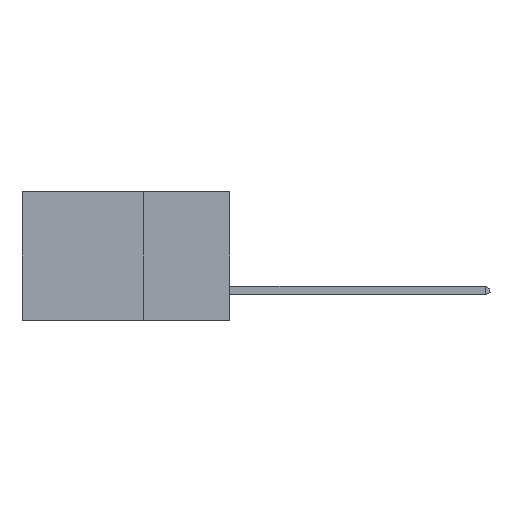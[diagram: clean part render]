
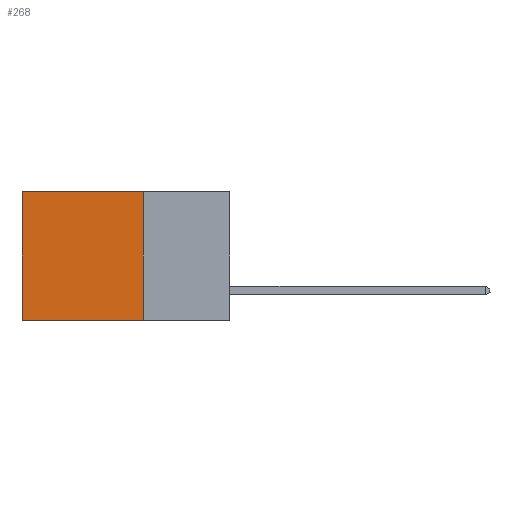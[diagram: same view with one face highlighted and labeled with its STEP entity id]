
A CAD part, left-side view. The second image highlights one B-rep face of the part: STEP entity #268.
In plain terms, the highlighted planar face has unit normal (-1, 0, 0).
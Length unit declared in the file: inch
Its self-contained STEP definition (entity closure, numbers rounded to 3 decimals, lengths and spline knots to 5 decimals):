
#268 = ADVANCED_FACE ( 'NONE', ( #10347 ), #14118, .F. ) ;
#783 = CARTESIAN_POINT ( 'NONE',  ( 0.298, 0.25, -0.37 ) ) ;
#1923 = CARTESIAN_POINT ( 'NONE',  ( 0.298, 0.6, 0. ) ) ;
#2103 = EDGE_CURVE ( 'NONE', #6059, #18060, #12095, .T. ) ;
#2586 = ORIENTED_EDGE ( 'NONE', *, *, #2103, .F. ) ;
#3015 = AXIS2_PLACEMENT_3D ( 'NONE', #20912, #3309, #9962 ) ;
#3309 = DIRECTION ( 'NONE',  ( 1., 0., 0. ) ) ;
#5392 = LINE ( 'NONE', #783, #20162 ) ;
#5785 = VERTEX_POINT ( 'NONE', #20310 ) ;
#6059 = VERTEX_POINT ( 'NONE', #13394 ) ;
#6519 = CARTESIAN_POINT ( 'NONE',  ( 0.298, 0.25, 0. ) ) ;
#6719 = CARTESIAN_POINT ( 'NONE',  ( 0.298, 0.25, 0. ) ) ;
#6841 = LINE ( 'NONE', #1923, #18785 ) ;
#9962 = DIRECTION ( 'NONE',  ( 0., 0., -1. ) ) ;
#10347 = FACE_OUTER_BOUND ( 'NONE', #27989, .T. ) ;
#10906 = ORIENTED_EDGE ( 'NONE', *, *, #12861, .F. ) ;
#12095 = LINE ( 'NONE', #6719, #21384 ) ;
#12435 = ORIENTED_EDGE ( 'NONE', *, *, #14252, .T. ) ;
#12861 = EDGE_CURVE ( 'NONE', #18060, #5785, #5392, .T. ) ;
#13394 = CARTESIAN_POINT ( 'NONE',  ( 0.298, 0.25, 0. ) ) ;
#13502 = CARTESIAN_POINT ( 'NONE',  ( 0.298, 0.25, -0.37 ) ) ;
#14118 = PLANE ( 'NONE',  #3015 ) ;
#14252 = EDGE_CURVE ( 'NONE', #6059, #21270, #27258, .T. ) ;
#14572 = CARTESIAN_POINT ( 'NONE',  ( 0.298, 0.6, 0. ) ) ;
#17313 = DIRECTION ( 'NONE',  ( 0., 0., -1. ) ) ;
#17530 = DIRECTION ( 'NONE',  ( 0., 0., -1. ) ) ;
#17904 = EDGE_CURVE ( 'NONE', #21270, #5785, #6841, .T. ) ;
#18060 = VERTEX_POINT ( 'NONE', #13502 ) ;
#18394 = DIRECTION ( 'NONE',  ( 0., 1., 0. ) ) ;
#18785 = VECTOR ( 'NONE', #17313, 39.37008 ) ;
#20162 = VECTOR ( 'NONE', #18394, 39.37008 ) ;
#20310 = CARTESIAN_POINT ( 'NONE',  ( 0.298, 0.6, -0.37 ) ) ;
#20912 = CARTESIAN_POINT ( 'NONE',  ( 0.298, 0.25, 0. ) ) ;
#21270 = VERTEX_POINT ( 'NONE', #14572 ) ;
#21384 = VECTOR ( 'NONE', #17530, 39.37008 ) ;
#25517 = ORIENTED_EDGE ( 'NONE', *, *, #17904, .T. ) ;
#26199 = DIRECTION ( 'NONE',  ( 0., 1., 0. ) ) ;
#26943 = VECTOR ( 'NONE', #26199, 39.37008 ) ;
#27258 = LINE ( 'NONE', #6519, #26943 ) ;
#27989 = EDGE_LOOP ( 'NONE', ( #25517, #10906, #2586, #12435 ) ) ;
